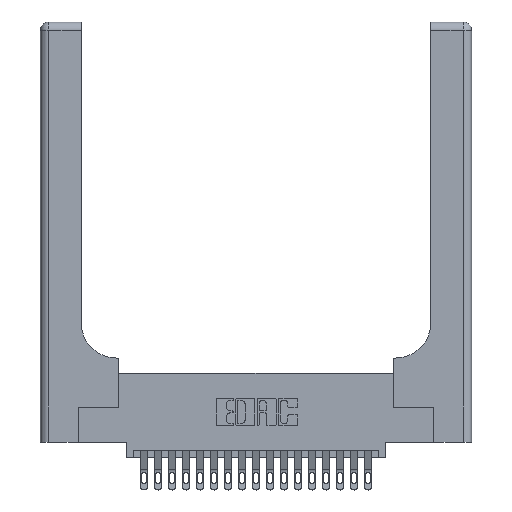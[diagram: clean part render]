
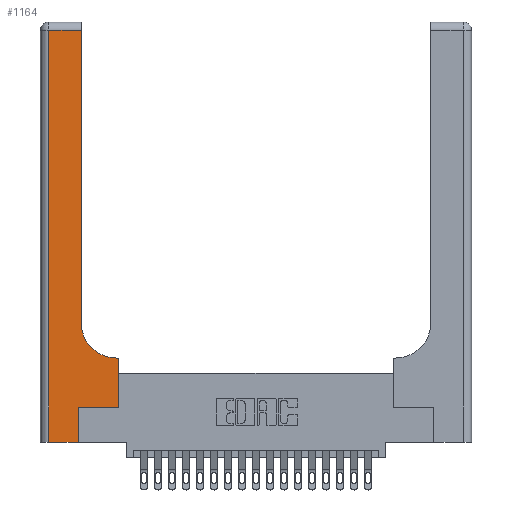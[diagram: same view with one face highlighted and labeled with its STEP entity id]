
A CAD part, top view. The second image highlights one B-rep face of the part: STEP entity #1164.
In plain terms, the highlighted planar face has unit normal (0, 0, 1).
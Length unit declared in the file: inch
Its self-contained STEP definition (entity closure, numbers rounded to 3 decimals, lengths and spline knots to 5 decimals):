
#295 = CARTESIAN_POINT ( 'NONE',  ( 0.5585, 0.6, 0.37 ) ) ;
#369 = LINE ( 'NONE', #5522, #4468 ) ;
#451 = DIRECTION ( 'NONE',  ( 1., 0., 0. ) ) ;
#1164 = ADVANCED_FACE ( 'NONE', ( #16094 ), #7124, .F. ) ;
#1648 = DIRECTION ( 'NONE',  ( 0., 1., 0. ) ) ;
#1762 = VERTEX_POINT ( 'NONE', #12267 ) ;
#2028 = DIRECTION ( 'NONE',  ( 1., 0., 0. ) ) ;
#2047 = VERTEX_POINT ( 'NONE', #4610 ) ;
#2204 = VERTEX_POINT ( 'NONE', #295 ) ;
#2825 = LINE ( 'NONE', #21126, #7450 ) ;
#3032 = CIRCLE ( 'NONE', #18617, 0.25 ) ;
#3271 = ORIENTED_EDGE ( 'NONE', *, *, #6547, .T. ) ;
#3911 = DIRECTION ( 'NONE',  ( 0., 0., -1. ) ) ;
#3942 = CARTESIAN_POINT ( 'NONE',  ( 0.5415, 0.6, 0.37 ) ) ;
#4333 = CARTESIAN_POINT ( 'NONE',  ( 0.269, 0., 0.37 ) ) ;
#4468 = VECTOR ( 'NONE', #2028, 39.37008 ) ;
#4528 = DIRECTION ( 'NONE',  ( -1., 0., 0. ) ) ;
#4610 = CARTESIAN_POINT ( 'NONE',  ( 0.5585, 0.25, 0.37 ) ) ;
#5192 = CARTESIAN_POINT ( 'NONE',  ( 0.2915, 3., 0.37 ) ) ;
#5522 = CARTESIAN_POINT ( 'NONE',  ( 0.269, 0.25, 0.37 ) ) ;
#6071 = CARTESIAN_POINT ( 'NONE',  ( 0.269, 0.25, 0.37 ) ) ;
#6149 = CARTESIAN_POINT ( 'NONE',  ( 0.06, 2.94, 0.37 ) ) ;
#6276 = VECTOR ( 'NONE', #13011, 39.37008 ) ;
#6547 = EDGE_CURVE ( 'NONE', #2204, #10667, #21895, .T. ) ;
#6589 = EDGE_CURVE ( 'NONE', #10667, #10102, #3032, .T. ) ;
#6950 = DIRECTION ( 'NONE',  ( 0., 1., 0. ) ) ;
#6989 = DIRECTION ( 'NONE',  ( 0., 0., -1. ) ) ;
#7039 = CARTESIAN_POINT ( 'NONE',  ( 0., 3., 0.37 ) ) ;
#7124 = PLANE ( 'NONE',  #10059 ) ;
#7160 = ORIENTED_EDGE ( 'NONE', *, *, #13164, .T. ) ;
#7276 = CARTESIAN_POINT ( 'NONE',  ( 0.2915, 0.6, 0.37 ) ) ;
#7450 = VECTOR ( 'NONE', #451, 39.37008 ) ;
#7787 = DIRECTION ( 'NONE',  ( 0., -1., 0. ) ) ;
#8208 = VECTOR ( 'NONE', #21015, 39.37008 ) ;
#8213 = CARTESIAN_POINT ( 'NONE',  ( 0.269, 0., 0.37 ) ) ;
#9189 = EDGE_CURVE ( 'NONE', #14546, #1762, #13515, .T. ) ;
#10059 = AXIS2_PLACEMENT_3D ( 'NONE', #7039, #6989, #17551 ) ;
#10102 = VERTEX_POINT ( 'NONE', #22081 ) ;
#10598 = EDGE_CURVE ( 'NONE', #16807, #14546, #21012, .T. ) ;
#10667 = VERTEX_POINT ( 'NONE', #3942 ) ;
#11168 = VECTOR ( 'NONE', #1648, 39.37008 ) ;
#11513 = ORIENTED_EDGE ( 'NONE', *, *, #10598, .T. ) ;
#11705 = LINE ( 'NONE', #13801, #11168 ) ;
#11749 = EDGE_CURVE ( 'NONE', #10102, #16807, #22314, .T. ) ;
#12267 = CARTESIAN_POINT ( 'NONE',  ( 0.06, 0., 0.37 ) ) ;
#13011 = DIRECTION ( 'NONE',  ( 0., 1., 0. ) ) ;
#13022 = EDGE_LOOP ( 'NONE', ( #15143, #11513, #17838, #16829, #13782, #7160, #20735, #3271, #13224 ) ) ;
#13164 = EDGE_CURVE ( 'NONE', #16279, #2047, #369, .T. ) ;
#13224 = ORIENTED_EDGE ( 'NONE', *, *, #6589, .T. ) ;
#13515 = LINE ( 'NONE', #19806, #22059 ) ;
#13782 = ORIENTED_EDGE ( 'NONE', *, *, #15635, .T. ) ;
#13801 = CARTESIAN_POINT ( 'NONE',  ( 0.5585, 0.25, 0.37 ) ) ;
#14317 = CARTESIAN_POINT ( 'NONE',  ( 0.5415, 0.85, 0.37 ) ) ;
#14546 = VERTEX_POINT ( 'NONE', #6149 ) ;
#14934 = CARTESIAN_POINT ( 'NONE',  ( 0., 2.94, 0.37 ) ) ;
#15143 = ORIENTED_EDGE ( 'NONE', *, *, #11749, .T. ) ;
#15635 = EDGE_CURVE ( 'NONE', #15746, #16279, #20002, .T. ) ;
#15746 = VERTEX_POINT ( 'NONE', #8213 ) ;
#16048 = DIRECTION ( 'NONE',  ( 1., 0., 0. ) ) ;
#16094 = FACE_OUTER_BOUND ( 'NONE', #13022, .T. ) ;
#16279 = VERTEX_POINT ( 'NONE', #6071 ) ;
#16807 = VERTEX_POINT ( 'NONE', #19506 ) ;
#16829 = ORIENTED_EDGE ( 'NONE', *, *, #19930, .T. ) ;
#17551 = DIRECTION ( 'NONE',  ( -1., 0., 0. ) ) ;
#17838 = ORIENTED_EDGE ( 'NONE', *, *, #9189, .T. ) ;
#18089 = VECTOR ( 'NONE', #4528, 39.37008 ) ;
#18182 = EDGE_CURVE ( 'NONE', #2047, #2204, #11705, .T. ) ;
#18617 = AXIS2_PLACEMENT_3D ( 'NONE', #14317, #3911, #16048 ) ;
#19506 = CARTESIAN_POINT ( 'NONE',  ( 0.2915, 2.94, 0.37 ) ) ;
#19806 = CARTESIAN_POINT ( 'NONE',  ( 0.06, 3., 0.37 ) ) ;
#19930 = EDGE_CURVE ( 'NONE', #1762, #15746, #2825, .T. ) ;
#20002 = LINE ( 'NONE', #4333, #6276 ) ;
#20735 = ORIENTED_EDGE ( 'NONE', *, *, #18182, .T. ) ;
#21012 = LINE ( 'NONE', #14934, #18089 ) ;
#21015 = DIRECTION ( 'NONE',  ( -1., 0., 0. ) ) ;
#21126 = CARTESIAN_POINT ( 'NONE',  ( 0., 0., 0.37 ) ) ;
#21769 = VECTOR ( 'NONE', #6950, 39.37008 ) ;
#21895 = LINE ( 'NONE', #7276, #8208 ) ;
#22059 = VECTOR ( 'NONE', #7787, 39.37008 ) ;
#22081 = CARTESIAN_POINT ( 'NONE',  ( 0.2915, 0.85, 0.37 ) ) ;
#22314 = LINE ( 'NONE', #5192, #21769 ) ;
